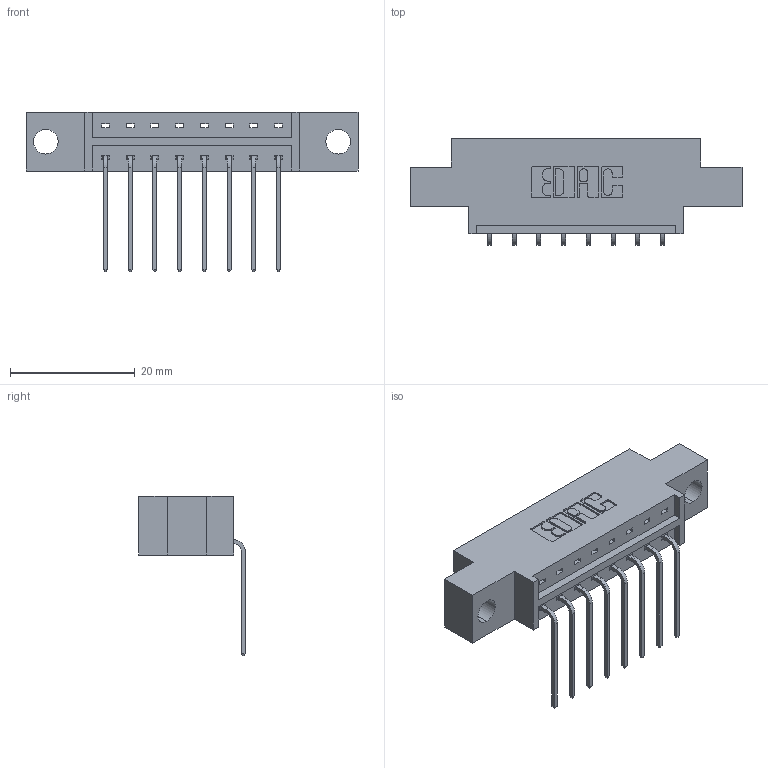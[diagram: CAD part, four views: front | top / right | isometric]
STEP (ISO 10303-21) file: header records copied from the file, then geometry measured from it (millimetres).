
FILE_DESCRIPTION (( 'STEP AP203' ), '1' );
FILE_NAME ('833-008-559-604.STEP', '2020-05-30T16:42:17', ( '' ), ( '' ), 'SwSTEP 2.0', 'SolidWorks 2020', '' );
FILE_SCHEMA (( 'CONFIG_CONTROL_DESIGN' ));
Length unit declared in the file: inch
Products named in the file (3): 833-008-559-604; 345-292-001_558 559 Tail - 1; 833 Part_Offset - .156 Dia - TH
Assembly tree (9 placements, depth 2):
  833-008-559-604
    833 Part_Offset - .156 Dia - TH
    345-292-001_558 559 Tail - 1  x8
Bounding box: 53.24 x 17.09 x 25.53 mm (x, y, z)
Volume: 4775.9 mm3; surface area: 5101.7 mm2
Topology: 9 solids, 9 shells, 598 faces, 1779 edges, 1174 vertices
Faces by surface type: plane 426, cylinder 172
Entity records: 9507 total; most frequent: CARTESIAN_POINT 1654, ORIENTED_EDGE 1598, DIRECTION 1463, EDGE_CURVE 799, VECTOR 671, LINE 671, VERTEX_POINT 530, AXIS2_PLACEMENT_3D 396
